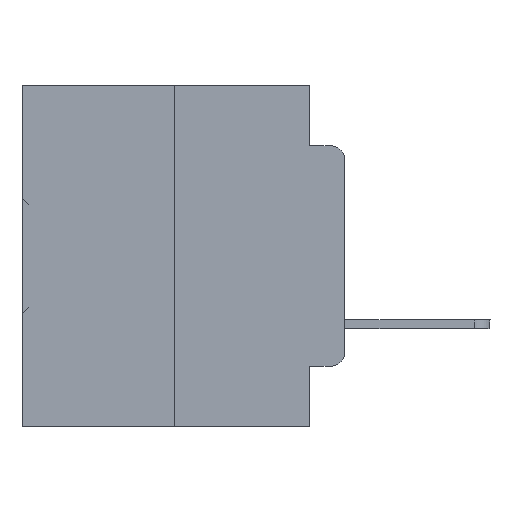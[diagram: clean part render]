
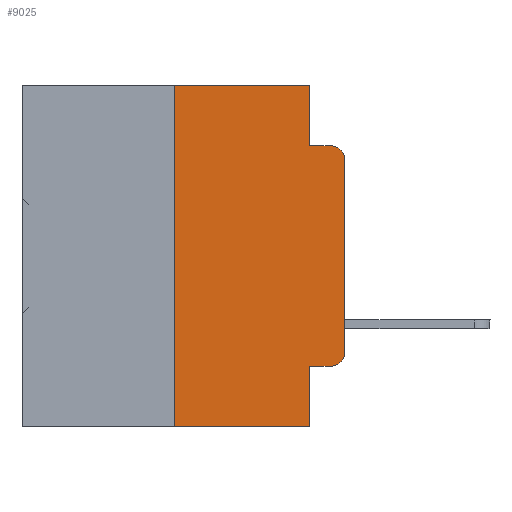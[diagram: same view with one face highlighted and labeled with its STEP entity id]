
A CAD part, left-side view. The second image highlights one B-rep face of the part: STEP entity #9025.
In plain terms, the highlighted planar face has unit normal (-1, 0, 0).
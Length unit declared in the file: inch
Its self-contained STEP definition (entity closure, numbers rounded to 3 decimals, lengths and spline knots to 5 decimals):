
#1127 = ORIENTED_EDGE ( 'NONE', *, *, #32524, .F. ) ;
#1375 = AXIS2_PLACEMENT_3D ( 'NONE', #29536, #30165, #7683 ) ;
#1488 = FACE_OUTER_BOUND ( 'NONE', #4162, .T. ) ;
#1536 = VERTEX_POINT ( 'NONE', #21563 ) ;
#1605 = CARTESIAN_POINT ( 'NONE',  ( 0., 0.051, -0.5 ) ) ;
#1726 = CARTESIAN_POINT ( 'NONE',  ( 0., 0.25, 0. ) ) ;
#1851 = EDGE_CURVE ( 'NONE', #22750, #32428, #20834, .T. ) ;
#1869 = VECTOR ( 'NONE', #32830, 39.37008 ) ;
#1885 = LINE ( 'NONE', #10253, #8875 ) ;
#2305 = AXIS2_PLACEMENT_3D ( 'NONE', #23964, #35211, #26812 ) ;
#2530 = EDGE_CURVE ( 'NONE', #8530, #8614, #19055, .T. ) ;
#2555 = LINE ( 'NONE', #31720, #24877 ) ;
#2602 = EDGE_CURVE ( 'NONE', #22892, #10292, #9415, .T. ) ;
#3351 = CARTESIAN_POINT ( 'NONE',  ( 0., 0., -0.3915 ) ) ;
#3815 = EDGE_CURVE ( 'NONE', #19085, #21263, #1885, .T. ) ;
#4162 = EDGE_LOOP ( 'NONE', ( #25643, #30074, #31383, #6384, #35007, #28752, #24605, #1127, #35720, #16643 ) ) ;
#6221 = CARTESIAN_POINT ( 'NONE',  ( 0., 0.051, 0. ) ) ;
#6384 = ORIENTED_EDGE ( 'NONE', *, *, #2530, .F. ) ;
#6524 = DIRECTION ( 'NONE',  ( 0., -1., 0. ) ) ;
#7683 = DIRECTION ( 'NONE',  ( 0., 0., -1. ) ) ;
#7689 = DIRECTION ( 'NONE',  ( 0., 0., 1. ) ) ;
#8530 = VERTEX_POINT ( 'NONE', #6221 ) ;
#8614 = VERTEX_POINT ( 'NONE', #12210 ) ;
#8875 = VECTOR ( 'NONE', #7689, 39.37008 ) ;
#9025 = ADVANCED_FACE ( 'NONE', ( #1488 ), #24201, .F. ) ;
#9415 = LINE ( 'NONE', #25554, #10741 ) ;
#9924 = CARTESIAN_POINT ( 'NONE',  ( 0., 0.473, -0.5 ) ) ;
#10253 = CARTESIAN_POINT ( 'NONE',  ( 0., 0., 0. ) ) ;
#10292 = VERTEX_POINT ( 'NONE', #29507 ) ;
#10359 = CARTESIAN_POINT ( 'NONE',  ( 0., 0.25, 0. ) ) ;
#10563 = LINE ( 'NONE', #24366, #14907 ) ;
#10741 = VECTOR ( 'NONE', #28409, 39.37008 ) ;
#12210 = CARTESIAN_POINT ( 'NONE',  ( 0., 0.051, -0.0885 ) ) ;
#12396 = CARTESIAN_POINT ( 'NONE',  ( 0., 0.02, -0.3915 ) ) ;
#12827 = DIRECTION ( 'NONE',  ( 0., 0., 1. ) ) ;
#13437 = VECTOR ( 'NONE', #32695, 39.37008 ) ;
#14401 = CARTESIAN_POINT ( 'NONE',  ( 0., 0.051, 0. ) ) ;
#14691 = EDGE_CURVE ( 'NONE', #30082, #8530, #24628, .T. ) ;
#14907 = VECTOR ( 'NONE', #27215, 39.37008 ) ;
#14982 = DIRECTION ( 'NONE',  ( 0., 0., -1. ) ) ;
#16643 = ORIENTED_EDGE ( 'NONE', *, *, #23396, .T. ) ;
#17199 = VECTOR ( 'NONE', #12827, 39.37008 ) ;
#18149 = VECTOR ( 'NONE', #19904, 39.37008 ) ;
#19055 = LINE ( 'NONE', #14401, #18149 ) ;
#19085 = VERTEX_POINT ( 'NONE', #3351 ) ;
#19904 = DIRECTION ( 'NONE',  ( 0., 0., -1. ) ) ;
#20400 = CIRCLE ( 'NONE', #2305, 0.02 ) ;
#20834 = LINE ( 'NONE', #9924, #13437 ) ;
#20946 = CARTESIAN_POINT ( 'NONE',  ( 0., 0., -0.1085 ) ) ;
#21263 = VERTEX_POINT ( 'NONE', #20946 ) ;
#21563 = CARTESIAN_POINT ( 'NONE',  ( 0., 0.02, -0.0885 ) ) ;
#22750 = VERTEX_POINT ( 'NONE', #28341 ) ;
#22854 = EDGE_CURVE ( 'NONE', #22750, #30082, #30477, .T. ) ;
#22892 = VERTEX_POINT ( 'NONE', #32170 ) ;
#23396 = EDGE_CURVE ( 'NONE', #10292, #19085, #30883, .T. ) ;
#23964 = CARTESIAN_POINT ( 'NONE',  ( 0., 0.02, -0.1085 ) ) ;
#24201 = PLANE ( 'NONE',  #1375 ) ;
#24366 = CARTESIAN_POINT ( 'NONE',  ( 0., 0.051, 0. ) ) ;
#24605 = ORIENTED_EDGE ( 'NONE', *, *, #1851, .T. ) ;
#24628 = LINE ( 'NONE', #27001, #1869 ) ;
#24877 = VECTOR ( 'NONE', #6524, 39.37008 ) ;
#25554 = CARTESIAN_POINT ( 'NONE',  ( 0., 0.051, -0.4115 ) ) ;
#25643 = ORIENTED_EDGE ( 'NONE', *, *, #3815, .T. ) ;
#26812 = DIRECTION ( 'NONE',  ( 0., 0., -1. ) ) ;
#27001 = CARTESIAN_POINT ( 'NONE',  ( 0., 0.473, 0. ) ) ;
#27215 = DIRECTION ( 'NONE',  ( 0., 0., -1. ) ) ;
#27515 = EDGE_CURVE ( 'NONE', #21263, #1536, #20400, .T. ) ;
#28341 = CARTESIAN_POINT ( 'NONE',  ( 0., 0.25, -0.5 ) ) ;
#28358 = EDGE_CURVE ( 'NONE', #8614, #1536, #2555, .T. ) ;
#28409 = DIRECTION ( 'NONE',  ( 0., -1., 0. ) ) ;
#28752 = ORIENTED_EDGE ( 'NONE', *, *, #22854, .F. ) ;
#29507 = CARTESIAN_POINT ( 'NONE',  ( 0., 0.02, -0.4115 ) ) ;
#29536 = CARTESIAN_POINT ( 'NONE',  ( 0., 0.473, 0. ) ) ;
#30074 = ORIENTED_EDGE ( 'NONE', *, *, #27515, .T. ) ;
#30082 = VERTEX_POINT ( 'NONE', #10359 ) ;
#30165 = DIRECTION ( 'NONE',  ( 1., 0., 0. ) ) ;
#30477 = LINE ( 'NONE', #1726, #17199 ) ;
#30883 = CIRCLE ( 'NONE', #33711, 0.02 ) ;
#31383 = ORIENTED_EDGE ( 'NONE', *, *, #28358, .F. ) ;
#31720 = CARTESIAN_POINT ( 'NONE',  ( 0., 0.051, -0.0885 ) ) ;
#31862 = DIRECTION ( 'NONE',  ( -1., 0., 0. ) ) ;
#32170 = CARTESIAN_POINT ( 'NONE',  ( 0., 0.051, -0.4115 ) ) ;
#32428 = VERTEX_POINT ( 'NONE', #1605 ) ;
#32524 = EDGE_CURVE ( 'NONE', #22892, #32428, #10563, .T. ) ;
#32695 = DIRECTION ( 'NONE',  ( 0., -1., 0. ) ) ;
#32830 = DIRECTION ( 'NONE',  ( 0., -1., 0. ) ) ;
#33711 = AXIS2_PLACEMENT_3D ( 'NONE', #12396, #31862, #14982 ) ;
#35007 = ORIENTED_EDGE ( 'NONE', *, *, #14691, .F. ) ;
#35211 = DIRECTION ( 'NONE',  ( -1., 0., 0. ) ) ;
#35720 = ORIENTED_EDGE ( 'NONE', *, *, #2602, .T. ) ;
